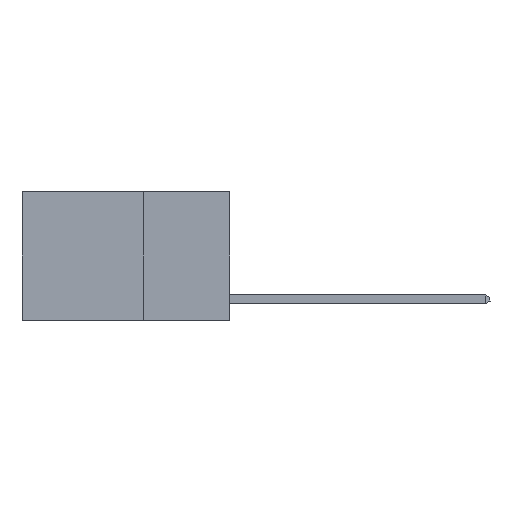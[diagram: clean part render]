
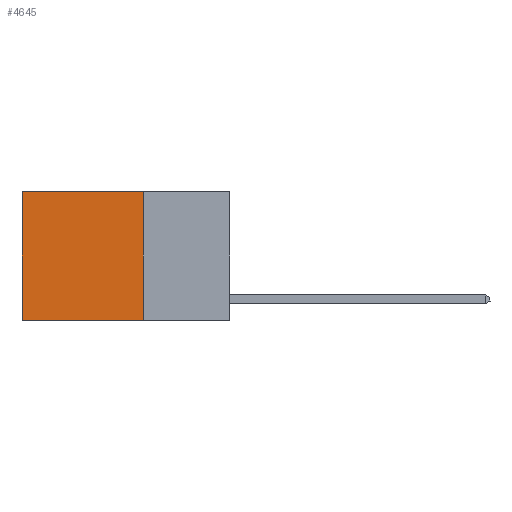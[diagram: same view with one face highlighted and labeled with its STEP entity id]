
A CAD part, left-side view. The second image highlights one B-rep face of the part: STEP entity #4645.
In plain terms, the highlighted planar face has unit normal (-1, 0, 0).
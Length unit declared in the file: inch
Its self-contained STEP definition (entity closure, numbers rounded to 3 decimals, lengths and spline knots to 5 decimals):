
#31 = CARTESIAN_POINT ( 'NONE',  ( 0.2625, 0.25, 0. ) ) ;
#1121 = EDGE_CURVE ( 'NONE', #16555, #2795, #16459, .T. ) ;
#1996 = DIRECTION ( 'NONE',  ( 0., 0., -1. ) ) ;
#2136 = CARTESIAN_POINT ( 'NONE',  ( 0.2625, 0.6, -0.37 ) ) ;
#2579 = EDGE_LOOP ( 'NONE', ( #6860, #19837, #6488, #14446 ) ) ;
#2754 = EDGE_CURVE ( 'NONE', #10069, #2795, #12339, .T. ) ;
#2795 = VERTEX_POINT ( 'NONE', #2136 ) ;
#4645 = ADVANCED_FACE ( 'NONE', ( #18452 ), #8197, .F. ) ;
#5278 = EDGE_CURVE ( 'NONE', #17344, #16555, #10529, .T. ) ;
#5921 = CARTESIAN_POINT ( 'NONE',  ( 0.2625, 0.25, 0. ) ) ;
#6488 = ORIENTED_EDGE ( 'NONE', *, *, #5278, .F. ) ;
#6860 = ORIENTED_EDGE ( 'NONE', *, *, #2754, .T. ) ;
#8117 = DIRECTION ( 'NONE',  ( 0., 0., -1. ) ) ;
#8187 = CARTESIAN_POINT ( 'NONE',  ( 0.2625, 0.6, 0. ) ) ;
#8188 = VECTOR ( 'NONE', #1996, 39.37008 ) ;
#8197 = PLANE ( 'NONE',  #9552 ) ;
#8317 = CARTESIAN_POINT ( 'NONE',  ( 0.2625, 0.25, -0.37 ) ) ;
#8721 = DIRECTION ( 'NONE',  ( 0., 1., 0. ) ) ;
#9552 = AXIS2_PLACEMENT_3D ( 'NONE', #14357, #18933, #9780 ) ;
#9556 = VECTOR ( 'NONE', #8117, 39.37008 ) ;
#9780 = DIRECTION ( 'NONE',  ( 0., 0., -1. ) ) ;
#10069 = VERTEX_POINT ( 'NONE', #8187 ) ;
#10529 = LINE ( 'NONE', #31, #9556 ) ;
#10679 = DIRECTION ( 'NONE',  ( 0., 1., 0. ) ) ;
#12339 = LINE ( 'NONE', #16104, #8188 ) ;
#12452 = VECTOR ( 'NONE', #10679, 39.37008 ) ;
#13601 = CARTESIAN_POINT ( 'NONE',  ( 0.2625, 0.25, -0.37 ) ) ;
#14357 = CARTESIAN_POINT ( 'NONE',  ( 0.2625, 0.25, 0. ) ) ;
#14446 = ORIENTED_EDGE ( 'NONE', *, *, #17341, .T. ) ;
#16104 = CARTESIAN_POINT ( 'NONE',  ( 0.2625, 0.6, 0. ) ) ;
#16459 = LINE ( 'NONE', #8317, #19966 ) ;
#16506 = LINE ( 'NONE', #18281, #12452 ) ;
#16555 = VERTEX_POINT ( 'NONE', #13601 ) ;
#17341 = EDGE_CURVE ( 'NONE', #17344, #10069, #16506, .T. ) ;
#17344 = VERTEX_POINT ( 'NONE', #5921 ) ;
#18281 = CARTESIAN_POINT ( 'NONE',  ( 0.2625, 0.25, 0. ) ) ;
#18452 = FACE_OUTER_BOUND ( 'NONE', #2579, .T. ) ;
#18933 = DIRECTION ( 'NONE',  ( 1., 0., 0. ) ) ;
#19837 = ORIENTED_EDGE ( 'NONE', *, *, #1121, .F. ) ;
#19966 = VECTOR ( 'NONE', #8721, 39.37008 ) ;
